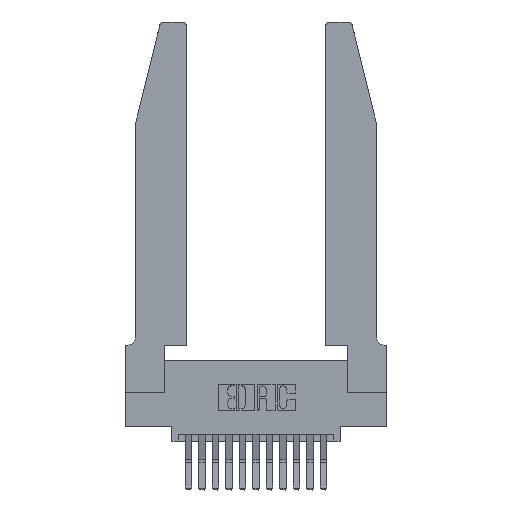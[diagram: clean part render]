
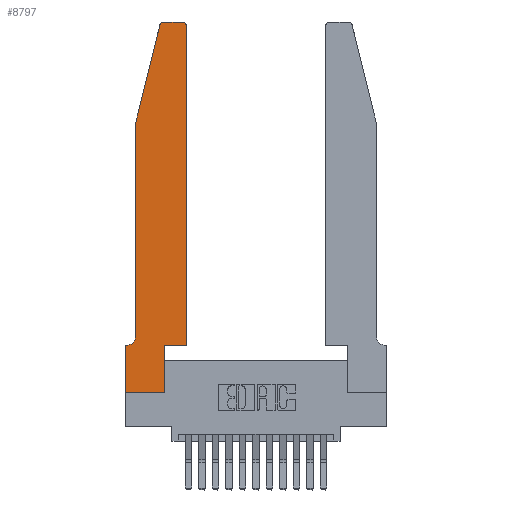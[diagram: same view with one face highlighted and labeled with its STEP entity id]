
A CAD part, top view. The second image highlights one B-rep face of the part: STEP entity #8797.
In plain terms, the highlighted planar face has unit normal (0, 0, 1).
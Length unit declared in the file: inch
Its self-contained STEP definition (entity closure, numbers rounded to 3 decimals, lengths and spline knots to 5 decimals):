
#117 = ORIENTED_EDGE ( 'NONE', *, *, #3430, .T. ) ;
#298 = VERTEX_POINT ( 'NONE', #6075 ) ;
#348 = VECTOR ( 'NONE', #11097, 39.37008 ) ;
#512 = VECTOR ( 'NONE', #7913, 39.37008 ) ;
#653 = DIRECTION ( 'NONE',  ( 1., 0., 0. ) ) ;
#820 = LINE ( 'NONE', #2820, #348 ) ;
#1003 = VERTEX_POINT ( 'NONE', #4710 ) ;
#1044 = DIRECTION ( 'NONE',  ( 0., 1., 0. ) ) ;
#1446 = LINE ( 'NONE', #16050, #512 ) ;
#1459 = VECTOR ( 'NONE', #10096, 39.37008 ) ;
#1611 = VERTEX_POINT ( 'NONE', #9335 ) ;
#1751 = CARTESIAN_POINT ( 'NONE',  ( 0.2865, 0., 0.37 ) ) ;
#1848 = CARTESIAN_POINT ( 'NONE',  ( 0.0755, 0.35, 0.37 ) ) ;
#1907 = CARTESIAN_POINT ( 'NONE',  ( 0., 0., 0.37 ) ) ;
#1919 = VERTEX_POINT ( 'NONE', #5979 ) ;
#2174 = EDGE_CURVE ( 'NONE', #15425, #5980, #4769, .T. ) ;
#2820 = CARTESIAN_POINT ( 'NONE',  ( 0.0755, 2., 0.37 ) ) ;
#2842 = AXIS2_PLACEMENT_3D ( 'NONE', #4327, #13955, #5724 ) ;
#3430 = EDGE_CURVE ( 'NONE', #1919, #5142, #12286, .T. ) ;
#3488 = CARTESIAN_POINT ( 'NONE',  ( 0.4505, 0.35, 0.37 ) ) ;
#3747 = VERTEX_POINT ( 'NONE', #6171 ) ;
#3881 = DIRECTION ( 'NONE',  ( 1., 0., 0. ) ) ;
#4070 = CARTESIAN_POINT ( 'NONE',  ( 0.4205, 2.72, 0.37 ) ) ;
#4138 = CARTESIAN_POINT ( 'NONE',  ( 0.2605, 2.75, 0.37 ) ) ;
#4327 = CARTESIAN_POINT ( 'NONE',  ( 0.284, 2.72, 0.37 ) ) ;
#4338 = ORIENTED_EDGE ( 'NONE', *, *, #9891, .T. ) ;
#4710 = CARTESIAN_POINT ( 'NONE',  ( 0.2865, 0.35, 0.37 ) ) ;
#4769 = LINE ( 'NONE', #4138, #12541 ) ;
#4801 = CARTESIAN_POINT ( 'NONE',  ( 0., 0., 0.37 ) ) ;
#5142 = VERTEX_POINT ( 'NONE', #6413 ) ;
#5271 = CARTESIAN_POINT ( 'NONE',  ( 0., 0.35, 0.37 ) ) ;
#5476 = DIRECTION ( 'NONE',  ( 1., 0., 0. ) ) ;
#5545 = VERTEX_POINT ( 'NONE', #1907 ) ;
#5724 = DIRECTION ( 'NONE',  ( 1., 0., 0. ) ) ;
#5979 = CARTESIAN_POINT ( 'NONE',  ( 0.0755, 0.42, 0.37 ) ) ;
#5980 = VERTEX_POINT ( 'NONE', #9776 ) ;
#6075 = CARTESIAN_POINT ( 'NONE',  ( 0., 0.35, 0.37 ) ) ;
#6171 = CARTESIAN_POINT ( 'NONE',  ( 0.25487, 2.72718, 0.37 ) ) ;
#6229 = ORIENTED_EDGE ( 'NONE', *, *, #14588, .T. ) ;
#6267 = CARTESIAN_POINT ( 'NONE',  ( 0.4505, 2.72, 0.37 ) ) ;
#6413 = CARTESIAN_POINT ( 'NONE',  ( 0.0055, 0.35, 0.37 ) ) ;
#6588 = EDGE_CURVE ( 'NONE', #3747, #1611, #820, .T. ) ;
#6660 = DIRECTION ( 'NONE',  ( 1., 0., 0. ) ) ;
#6745 = LINE ( 'NONE', #17455, #17123 ) ;
#6896 = CIRCLE ( 'NONE', #2842, 0.03 ) ;
#7219 = ORIENTED_EDGE ( 'NONE', *, *, #2174, .T. ) ;
#7307 = LINE ( 'NONE', #10767, #11392 ) ;
#7404 = EDGE_CURVE ( 'NONE', #5142, #298, #13226, .T. ) ;
#7478 = VECTOR ( 'NONE', #653, 39.37008 ) ;
#7913 = DIRECTION ( 'NONE',  ( 0., 1., 0. ) ) ;
#8131 = ORIENTED_EDGE ( 'NONE', *, *, #15469, .T. ) ;
#8235 = CARTESIAN_POINT ( 'NONE',  ( 0.0055, 0.42, 0.37 ) ) ;
#8282 = DIRECTION ( 'NONE',  ( -1., 0., 0. ) ) ;
#8359 = LINE ( 'NONE', #4801, #14794 ) ;
#8459 = ORIENTED_EDGE ( 'NONE', *, *, #6588, .T. ) ;
#8696 = CARTESIAN_POINT ( 'NONE',  ( 0.0755, 2., 0.37 ) ) ;
#8797 = ADVANCED_FACE ( 'NONE', ( #15855 ), #9341, .T. ) ;
#8925 = DIRECTION ( 'NONE',  ( 0., -1., 0. ) ) ;
#9089 = VECTOR ( 'NONE', #11485, 39.37008 ) ;
#9156 = CARTESIAN_POINT ( 'NONE',  ( 0.4205, 2.75, 0.37 ) ) ;
#9335 = CARTESIAN_POINT ( 'NONE',  ( 0.0755, 2., 0.37 ) ) ;
#9341 = PLANE ( 'NONE',  #10001 ) ;
#9428 = EDGE_CURVE ( 'NONE', #5980, #3747, #6896, .T. ) ;
#9622 = DIRECTION ( 'NONE',  ( -1., 0., 0. ) ) ;
#9776 = CARTESIAN_POINT ( 'NONE',  ( 0.284, 2.75, 0.37 ) ) ;
#9886 = ORIENTED_EDGE ( 'NONE', *, *, #14263, .T. ) ;
#9891 = EDGE_CURVE ( 'NONE', #5545, #12516, #7307, .T. ) ;
#9966 = ORIENTED_EDGE ( 'NONE', *, *, #11009, .T. ) ;
#10001 = AXIS2_PLACEMENT_3D ( 'NONE', #5271, #14832, #6660 ) ;
#10096 = DIRECTION ( 'NONE',  ( 0., -1., 0. ) ) ;
#10767 = CARTESIAN_POINT ( 'NONE',  ( 0., 0., 0.37 ) ) ;
#11009 = EDGE_CURVE ( 'NONE', #1003, #15589, #11135, .T. ) ;
#11097 = DIRECTION ( 'NONE',  ( -0.239, -0.971, 0. ) ) ;
#11135 = LINE ( 'NONE', #3488, #7478 ) ;
#11392 = VECTOR ( 'NONE', #3881, 39.37008 ) ;
#11485 = DIRECTION ( 'NONE',  ( -1., 0., 0. ) ) ;
#11986 = VERTEX_POINT ( 'NONE', #6267 ) ;
#12286 = CIRCLE ( 'NONE', #14867, 0.07 ) ;
#12516 = VERTEX_POINT ( 'NONE', #1751 ) ;
#12530 = ORIENTED_EDGE ( 'NONE', *, *, #9428, .T. ) ;
#12541 = VECTOR ( 'NONE', #8282, 39.37008 ) ;
#12568 = EDGE_LOOP ( 'NONE', ( #7219, #12530, #8459, #6229, #117, #12884, #12965, #4338, #8131, #9966, #9886, #15181 ) ) ;
#12884 = ORIENTED_EDGE ( 'NONE', *, *, #7404, .T. ) ;
#12889 = CIRCLE ( 'NONE', #14650, 0.03 ) ;
#12965 = ORIENTED_EDGE ( 'NONE', *, *, #16399, .T. ) ;
#13226 = LINE ( 'NONE', #1848, #9089 ) ;
#13722 = DIRECTION ( 'NONE',  ( 0., 0., 1. ) ) ;
#13955 = DIRECTION ( 'NONE',  ( 0., 0., 1. ) ) ;
#14263 = EDGE_CURVE ( 'NONE', #15589, #11986, #6745, .T. ) ;
#14588 = EDGE_CURVE ( 'NONE', #1611, #1919, #16082, .T. ) ;
#14650 = AXIS2_PLACEMENT_3D ( 'NONE', #4070, #13722, #5476 ) ;
#14794 = VECTOR ( 'NONE', #8925, 39.37008 ) ;
#14832 = DIRECTION ( 'NONE',  ( 0., 0., 1. ) ) ;
#14867 = AXIS2_PLACEMENT_3D ( 'NONE', #8235, #17684, #9622 ) ;
#15181 = ORIENTED_EDGE ( 'NONE', *, *, #17679, .T. ) ;
#15219 = CARTESIAN_POINT ( 'NONE',  ( 0.4505, 0.35, 0.37 ) ) ;
#15425 = VERTEX_POINT ( 'NONE', #9156 ) ;
#15469 = EDGE_CURVE ( 'NONE', #12516, #1003, #1446, .T. ) ;
#15589 = VERTEX_POINT ( 'NONE', #15219 ) ;
#15855 = FACE_OUTER_BOUND ( 'NONE', #12568, .T. ) ;
#16050 = CARTESIAN_POINT ( 'NONE',  ( 0.2865, 0.35, 0.37 ) ) ;
#16082 = LINE ( 'NONE', #8696, #1459 ) ;
#16399 = EDGE_CURVE ( 'NONE', #298, #5545, #8359, .T. ) ;
#17123 = VECTOR ( 'NONE', #1044, 39.37008 ) ;
#17455 = CARTESIAN_POINT ( 'NONE',  ( 0.4505, 0.35, 0.37 ) ) ;
#17679 = EDGE_CURVE ( 'NONE', #11986, #15425, #12889, .T. ) ;
#17684 = DIRECTION ( 'NONE',  ( 0., 0., -1. ) ) ;
